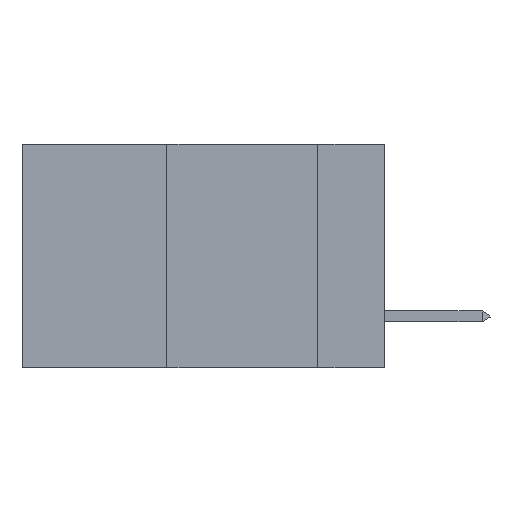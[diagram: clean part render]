
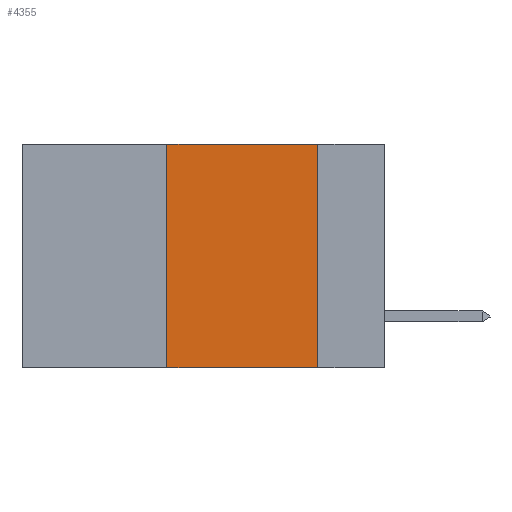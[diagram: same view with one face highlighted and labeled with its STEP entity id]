
A CAD part, left-side view. The second image highlights one B-rep face of the part: STEP entity #4355.
In plain terms, the highlighted planar face has unit normal (-1, 0, 0).
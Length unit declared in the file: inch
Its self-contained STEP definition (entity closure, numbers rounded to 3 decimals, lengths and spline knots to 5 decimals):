
#104 = LINE ( 'NONE', #32814, #549 ) ;
#549 = VECTOR ( 'NONE', #24872, 39.37008 ) ;
#941 = VERTEX_POINT ( 'NONE', #31972 ) ;
#2285 = CARTESIAN_POINT ( 'NONE',  ( 0., 0.11, 0. ) ) ;
#2891 = ORIENTED_EDGE ( 'NONE', *, *, #24624, .F. ) ;
#3551 = LINE ( 'NONE', #23349, #27054 ) ;
#4355 = ADVANCED_FACE ( 'NONE', ( #32744 ), #16232, .F. ) ;
#5162 = DIRECTION ( 'NONE',  ( 1., 0., 0. ) ) ;
#6454 = ORIENTED_EDGE ( 'NONE', *, *, #25426, .F. ) ;
#6623 = AXIS2_PLACEMENT_3D ( 'NONE', #16713, #5162, #19026 ) ;
#6841 = LINE ( 'NONE', #27189, #19496 ) ;
#9849 = EDGE_LOOP ( 'NONE', ( #25945, #6454, #2891, #24998 ) ) ;
#12441 = VERTEX_POINT ( 'NONE', #31372 ) ;
#12734 = VECTOR ( 'NONE', #33259, 39.37008 ) ;
#13614 = LINE ( 'NONE', #2285, #12734 ) ;
#16232 = PLANE ( 'NONE',  #6623 ) ;
#16713 = CARTESIAN_POINT ( 'NONE',  ( 0., 0.6, 0. ) ) ;
#17686 = EDGE_CURVE ( 'NONE', #12441, #35684, #6841, .T. ) ;
#18036 = VERTEX_POINT ( 'NONE', #28637 ) ;
#19026 = DIRECTION ( 'NONE',  ( 0., 0., -1. ) ) ;
#19496 = VECTOR ( 'NONE', #24020, 39.37008 ) ;
#23232 = DIRECTION ( 'NONE',  ( 0., -1., 0. ) ) ;
#23349 = CARTESIAN_POINT ( 'NONE',  ( 0., 0.6, 0. ) ) ;
#24020 = DIRECTION ( 'NONE',  ( 0., -1., 0. ) ) ;
#24624 = EDGE_CURVE ( 'NONE', #12441, #941, #104, .T. ) ;
#24872 = DIRECTION ( 'NONE',  ( 0., 0., 1. ) ) ;
#24998 = ORIENTED_EDGE ( 'NONE', *, *, #17686, .T. ) ;
#25426 = EDGE_CURVE ( 'NONE', #941, #18036, #3551, .T. ) ;
#25945 = ORIENTED_EDGE ( 'NONE', *, *, #31853, .F. ) ;
#27054 = VECTOR ( 'NONE', #23232, 39.37008 ) ;
#27189 = CARTESIAN_POINT ( 'NONE',  ( 0., 0.6, -0.37 ) ) ;
#28637 = CARTESIAN_POINT ( 'NONE',  ( 0., 0.11, 0. ) ) ;
#31372 = CARTESIAN_POINT ( 'NONE',  ( 0., 0.36, -0.37 ) ) ;
#31516 = CARTESIAN_POINT ( 'NONE',  ( 0., 0.11, -0.37 ) ) ;
#31853 = EDGE_CURVE ( 'NONE', #18036, #35684, #13614, .T. ) ;
#31972 = CARTESIAN_POINT ( 'NONE',  ( 0., 0.36, 0. ) ) ;
#32744 = FACE_OUTER_BOUND ( 'NONE', #9849, .T. ) ;
#32814 = CARTESIAN_POINT ( 'NONE',  ( 0., 0.36, 0. ) ) ;
#33259 = DIRECTION ( 'NONE',  ( 0., 0., -1. ) ) ;
#35684 = VERTEX_POINT ( 'NONE', #31516 ) ;
